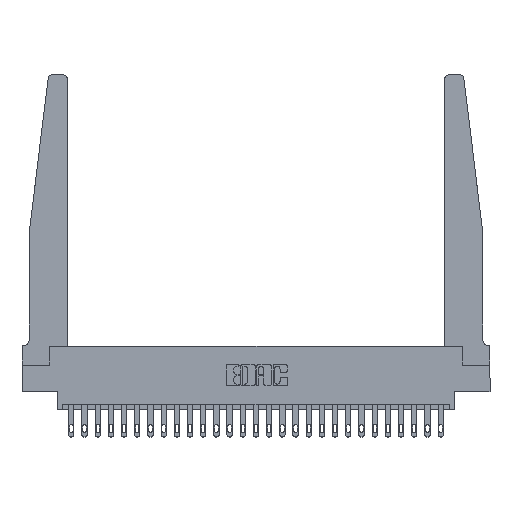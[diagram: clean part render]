
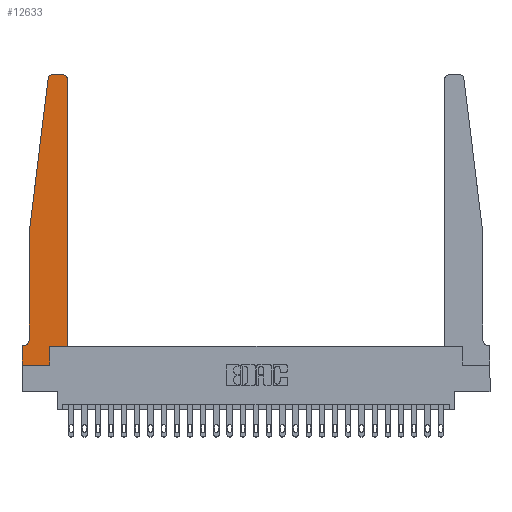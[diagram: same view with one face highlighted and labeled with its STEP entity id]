
A CAD part, top view. The second image highlights one B-rep face of the part: STEP entity #12633.
In plain terms, the highlighted planar face has unit normal (0, 0, 1).
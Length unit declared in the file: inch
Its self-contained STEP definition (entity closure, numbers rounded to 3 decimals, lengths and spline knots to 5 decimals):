
#181 = DIRECTION ( 'NONE',  ( 0., -1., 0. ) ) ;
#336 = DIRECTION ( 'NONE',  ( 0., 0., -1. ) ) ;
#531 = VERTEX_POINT ( 'NONE', #20125 ) ;
#828 = CARTESIAN_POINT ( 'NONE',  ( 0., 0.1875, 0.37 ) ) ;
#1045 = CARTESIAN_POINT ( 'NONE',  ( 0., 0., 0.37 ) ) ;
#1069 = CARTESIAN_POINT ( 'NONE',  ( 0.2605, 0.18, 0.37 ) ) ;
#1113 = EDGE_CURVE ( 'NONE', #13593, #531, #10971, .T. ) ;
#1530 = DIRECTION ( 'NONE',  ( 0., 1., 0. ) ) ;
#1547 = VERTEX_POINT ( 'NONE', #828 ) ;
#1739 = ORIENTED_EDGE ( 'NONE', *, *, #13048, .T. ) ;
#2070 = VECTOR ( 'NONE', #1530, 39.37008 ) ;
#2119 = DIRECTION ( 'NONE',  ( -0.122, -0.992, 0. ) ) ;
#2382 = LINE ( 'NONE', #6185, #8189 ) ;
#2486 = ORIENTED_EDGE ( 'NONE', *, *, #4882, .T. ) ;
#2708 = ORIENTED_EDGE ( 'NONE', *, *, #2731, .T. ) ;
#2731 = EDGE_CURVE ( 'NONE', #19815, #15734, #16858, .T. ) ;
#3288 = DIRECTION ( 'NONE',  ( 0., 0., 1. ) ) ;
#3750 = EDGE_CURVE ( 'NONE', #6625, #9715, #14379, .T. ) ;
#4070 = VERTEX_POINT ( 'NONE', #1069 ) ;
#4113 = LINE ( 'NONE', #6098, #16507 ) ;
#4319 = AXIS2_PLACEMENT_3D ( 'NONE', #5711, #21767, #22410 ) ;
#4510 = LINE ( 'NONE', #12567, #13337 ) ;
#4697 = ORIENTED_EDGE ( 'NONE', *, *, #15695, .T. ) ;
#4882 = EDGE_CURVE ( 'NONE', #9715, #14987, #8191, .T. ) ;
#4934 = CARTESIAN_POINT ( 'NONE',  ( 0.2605, 0., 0.37 ) ) ;
#4976 = CARTESIAN_POINT ( 'NONE',  ( 0.425, 2.72, 0.37 ) ) ;
#4990 = VECTOR ( 'NONE', #25346, 39.37008 ) ;
#5089 = EDGE_CURVE ( 'NONE', #11879, #13593, #4510, .T. ) ;
#5549 = VECTOR ( 'NONE', #22363, 39.37008 ) ;
#5711 = CARTESIAN_POINT ( 'NONE',  ( 0.395, 2.72, 0.37 ) ) ;
#5961 = DIRECTION ( 'NONE',  ( -1., 0., 0. ) ) ;
#6098 = CARTESIAN_POINT ( 'NONE',  ( 0.065, 0.1875, 0.37 ) ) ;
#6185 = CARTESIAN_POINT ( 'NONE',  ( 0.065, 1.25, 0.37 ) ) ;
#6188 = CARTESIAN_POINT ( 'NONE',  ( 0., 0., 0.37 ) ) ;
#6625 = VERTEX_POINT ( 'NONE', #24638 ) ;
#7046 = VECTOR ( 'NONE', #25778, 39.37008 ) ;
#7168 = DIRECTION ( 'NONE',  ( 0., 0., 1. ) ) ;
#7362 = ORIENTED_EDGE ( 'NONE', *, *, #20331, .T. ) ;
#7498 = CARTESIAN_POINT ( 'NONE',  ( 0., 0.1875, 0.37 ) ) ;
#7588 = CARTESIAN_POINT ( 'NONE',  ( 0.065, 1.25, 0.37 ) ) ;
#7915 = CARTESIAN_POINT ( 'NONE',  ( 0., 0., 0.37 ) ) ;
#8079 = ORIENTED_EDGE ( 'NONE', *, *, #22401, .T. ) ;
#8189 = VECTOR ( 'NONE', #2119, 39.37008 ) ;
#8191 = CIRCLE ( 'NONE', #19581, 0.03 ) ;
#8226 = VECTOR ( 'NONE', #24843, 39.37008 ) ;
#8931 = LINE ( 'NONE', #23127, #18136 ) ;
#9715 = VERTEX_POINT ( 'NONE', #11740 ) ;
#10339 = CARTESIAN_POINT ( 'NONE',  ( 0.015, 0.2375, 0.37 ) ) ;
#10394 = ORIENTED_EDGE ( 'NONE', *, *, #11017, .T. ) ;
#10671 = CARTESIAN_POINT ( 'NONE',  ( 0.425, 0.18, 0.37 ) ) ;
#10971 = CIRCLE ( 'NONE', #17705, 0.05 ) ;
#11017 = EDGE_CURVE ( 'NONE', #1547, #14989, #14123, .T. ) ;
#11200 = FACE_OUTER_BOUND ( 'NONE', #12057, .T. ) ;
#11740 = CARTESIAN_POINT ( 'NONE',  ( 0.27653, 2.75, 0.37 ) ) ;
#11743 = ORIENTED_EDGE ( 'NONE', *, *, #19077, .T. ) ;
#11869 = CARTESIAN_POINT ( 'NONE',  ( 0.25, 2.75, 0.37 ) ) ;
#11879 = VERTEX_POINT ( 'NONE', #7588 ) ;
#12057 = EDGE_LOOP ( 'NONE', ( #18745, #2486, #8079, #19262, #24757, #11743, #10394, #1739, #23677, #4697, #2708, #7362 ) ) ;
#12567 = CARTESIAN_POINT ( 'NONE',  ( 0.065, 1.25, 0.37 ) ) ;
#12633 = ADVANCED_FACE ( 'NONE', ( #11200 ), #25246, .T. ) ;
#13048 = EDGE_CURVE ( 'NONE', #14989, #13497, #19075, .T. ) ;
#13337 = VECTOR ( 'NONE', #181, 39.37008 ) ;
#13417 = AXIS2_PLACEMENT_3D ( 'NONE', #7498, #3288, #19231 ) ;
#13497 = VERTEX_POINT ( 'NONE', #4934 ) ;
#13529 = EDGE_CURVE ( 'NONE', #13497, #4070, #19424, .T. ) ;
#13593 = VERTEX_POINT ( 'NONE', #19680 ) ;
#14123 = LINE ( 'NONE', #6188, #7046 ) ;
#14379 = LINE ( 'NONE', #11869, #5549 ) ;
#14962 = DIRECTION ( 'NONE',  ( 1., 0., 0. ) ) ;
#14987 = VERTEX_POINT ( 'NONE', #15851 ) ;
#14989 = VERTEX_POINT ( 'NONE', #7915 ) ;
#15695 = EDGE_CURVE ( 'NONE', #4070, #19815, #8931, .T. ) ;
#15734 = VERTEX_POINT ( 'NONE', #4976 ) ;
#15851 = CARTESIAN_POINT ( 'NONE',  ( 0.24675, 2.72367, 0.37 ) ) ;
#16507 = VECTOR ( 'NONE', #5961, 39.37008 ) ;
#16844 = DIRECTION ( 'NONE',  ( 1., 0., 0. ) ) ;
#16858 = LINE ( 'NONE', #10671, #8226 ) ;
#16980 = CIRCLE ( 'NONE', #4319, 0.03 ) ;
#17192 = CARTESIAN_POINT ( 'NONE',  ( 0.27653, 2.72, 0.37 ) ) ;
#17705 = AXIS2_PLACEMENT_3D ( 'NONE', #10339, #336, #18497 ) ;
#17749 = CARTESIAN_POINT ( 'NONE',  ( 0.425, 0.18, 0.37 ) ) ;
#18136 = VECTOR ( 'NONE', #16844, 39.37008 ) ;
#18497 = DIRECTION ( 'NONE',  ( -1., 0., 0. ) ) ;
#18745 = ORIENTED_EDGE ( 'NONE', *, *, #3750, .T. ) ;
#19075 = LINE ( 'NONE', #1045, #4990 ) ;
#19077 = EDGE_CURVE ( 'NONE', #531, #1547, #4113, .T. ) ;
#19231 = DIRECTION ( 'NONE',  ( 1., 0., 0. ) ) ;
#19262 = ORIENTED_EDGE ( 'NONE', *, *, #5089, .T. ) ;
#19424 = LINE ( 'NONE', #23355, #2070 ) ;
#19581 = AXIS2_PLACEMENT_3D ( 'NONE', #17192, #7168, #14962 ) ;
#19680 = CARTESIAN_POINT ( 'NONE',  ( 0.065, 0.2375, 0.37 ) ) ;
#19815 = VERTEX_POINT ( 'NONE', #17749 ) ;
#20125 = CARTESIAN_POINT ( 'NONE',  ( 0.015, 0.1875, 0.37 ) ) ;
#20331 = EDGE_CURVE ( 'NONE', #15734, #6625, #16980, .T. ) ;
#21767 = DIRECTION ( 'NONE',  ( 0., 0., 1. ) ) ;
#22363 = DIRECTION ( 'NONE',  ( -1., 0., 0. ) ) ;
#22401 = EDGE_CURVE ( 'NONE', #14987, #11879, #2382, .T. ) ;
#22410 = DIRECTION ( 'NONE',  ( 1., 0., 0. ) ) ;
#23127 = CARTESIAN_POINT ( 'NONE',  ( 0.425, 0.18, 0.37 ) ) ;
#23355 = CARTESIAN_POINT ( 'NONE',  ( 0.2605, 0.18, 0.37 ) ) ;
#23677 = ORIENTED_EDGE ( 'NONE', *, *, #13529, .T. ) ;
#24638 = CARTESIAN_POINT ( 'NONE',  ( 0.395, 2.75, 0.37 ) ) ;
#24757 = ORIENTED_EDGE ( 'NONE', *, *, #1113, .T. ) ;
#24843 = DIRECTION ( 'NONE',  ( 0., 1., 0. ) ) ;
#25246 = PLANE ( 'NONE',  #13417 ) ;
#25346 = DIRECTION ( 'NONE',  ( 1., 0., 0. ) ) ;
#25778 = DIRECTION ( 'NONE',  ( 0., -1., 0. ) ) ;
